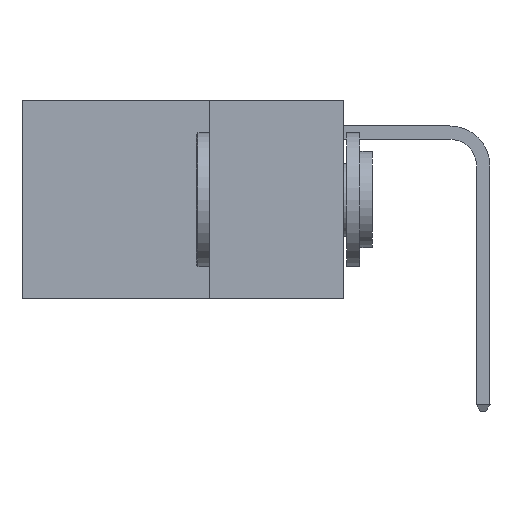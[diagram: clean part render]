
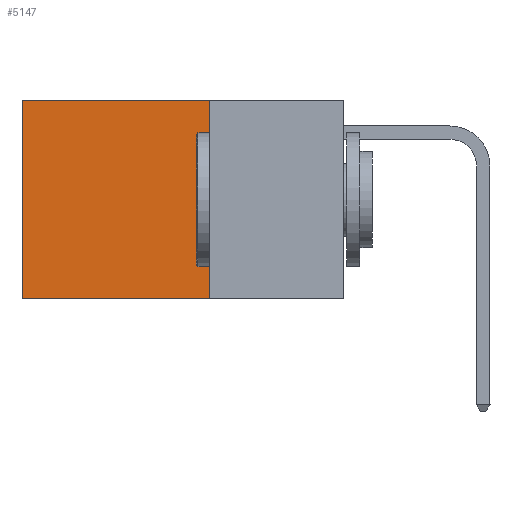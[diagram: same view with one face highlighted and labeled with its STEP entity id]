
A CAD part, left-side view. The second image highlights one B-rep face of the part: STEP entity #5147.
In plain terms, the highlighted planar face has unit normal (-1, 0, 0).
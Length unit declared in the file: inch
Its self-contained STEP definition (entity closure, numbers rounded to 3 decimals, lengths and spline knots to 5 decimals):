
#1163 = VECTOR ( 'NONE', #26777, 39.37008 ) ;
#1640 = ORIENTED_EDGE ( 'NONE', *, *, #2259, .T. ) ;
#1735 = EDGE_LOOP ( 'NONE', ( #1640, #4345, #9955, #8992 ) ) ;
#2138 = CARTESIAN_POINT ( 'NONE',  ( 0.2625, 0.25, -0.37 ) ) ;
#2259 = EDGE_CURVE ( 'NONE', #22926, #19755, #4641, .T. ) ;
#3589 = VECTOR ( 'NONE', #17331, 39.37008 ) ;
#4345 = ORIENTED_EDGE ( 'NONE', *, *, #19436, .F. ) ;
#4641 = LINE ( 'NONE', #16428, #26028 ) ;
#5147 = ADVANCED_FACE ( 'NONE', ( #16322 ), #25201, .F. ) ;
#5486 = AXIS2_PLACEMENT_3D ( 'NONE', #16904, #18632, #14296 ) ;
#5590 = VERTEX_POINT ( 'NONE', #2138 ) ;
#8010 = CARTESIAN_POINT ( 'NONE',  ( 0.2625, 0.25, 0. ) ) ;
#8220 = EDGE_CURVE ( 'NONE', #16362, #5590, #12967, .T. ) ;
#8992 = ORIENTED_EDGE ( 'NONE', *, *, #9695, .T. ) ;
#9695 = EDGE_CURVE ( 'NONE', #16362, #22926, #28667, .T. ) ;
#9955 = ORIENTED_EDGE ( 'NONE', *, *, #8220, .F. ) ;
#10387 = CARTESIAN_POINT ( 'NONE',  ( 0.2625, 0.6, -0.37 ) ) ;
#11276 = CARTESIAN_POINT ( 'NONE',  ( 0.2625, 0.25, -0.37 ) ) ;
#12776 = VECTOR ( 'NONE', #17810, 39.37008 ) ;
#12967 = LINE ( 'NONE', #8010, #3589 ) ;
#14114 = DIRECTION ( 'NONE',  ( 0., 0., -1. ) ) ;
#14296 = DIRECTION ( 'NONE',  ( 0., 0., -1. ) ) ;
#15685 = CARTESIAN_POINT ( 'NONE',  ( 0.2625, 0.6, 0. ) ) ;
#16322 = FACE_OUTER_BOUND ( 'NONE', #1735, .T. ) ;
#16362 = VERTEX_POINT ( 'NONE', #24480 ) ;
#16428 = CARTESIAN_POINT ( 'NONE',  ( 0.2625, 0.6, 0. ) ) ;
#16904 = CARTESIAN_POINT ( 'NONE',  ( 0.2625, 0.25, 0. ) ) ;
#17331 = DIRECTION ( 'NONE',  ( 0., 0., -1. ) ) ;
#17810 = DIRECTION ( 'NONE',  ( 0., 1., 0. ) ) ;
#18632 = DIRECTION ( 'NONE',  ( 1., 0., 0. ) ) ;
#19436 = EDGE_CURVE ( 'NONE', #5590, #19755, #26542, .T. ) ;
#19755 = VERTEX_POINT ( 'NONE', #10387 ) ;
#22926 = VERTEX_POINT ( 'NONE', #15685 ) ;
#24480 = CARTESIAN_POINT ( 'NONE',  ( 0.2625, 0.25, 0. ) ) ;
#24596 = CARTESIAN_POINT ( 'NONE',  ( 0.2625, 0.25, 0. ) ) ;
#25201 = PLANE ( 'NONE',  #5486 ) ;
#26028 = VECTOR ( 'NONE', #14114, 39.37008 ) ;
#26542 = LINE ( 'NONE', #11276, #12776 ) ;
#26777 = DIRECTION ( 'NONE',  ( 0., 1., 0. ) ) ;
#28667 = LINE ( 'NONE', #24596, #1163 ) ;
